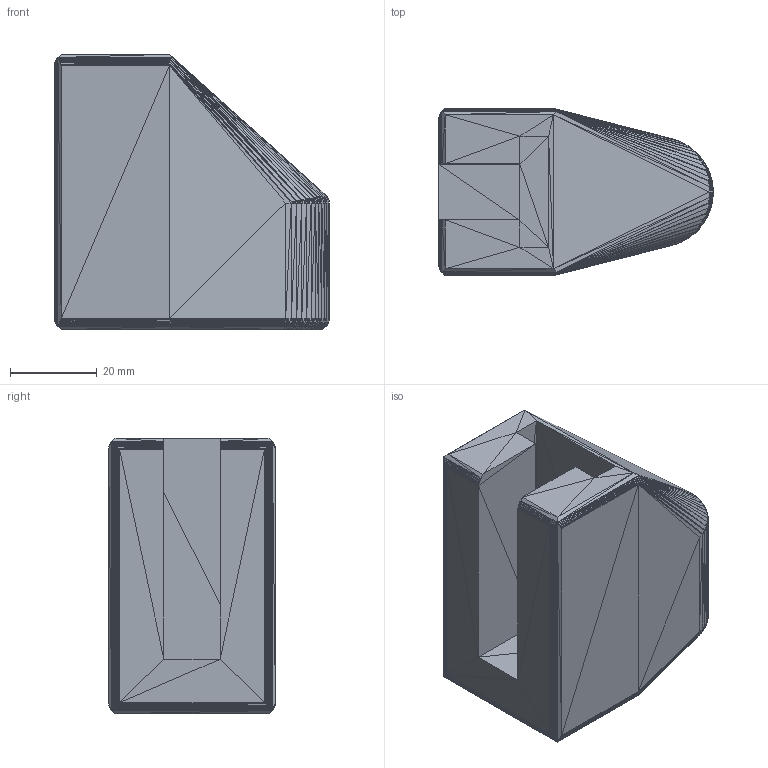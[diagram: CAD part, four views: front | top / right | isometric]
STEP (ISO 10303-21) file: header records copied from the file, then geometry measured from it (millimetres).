
FILE_DESCRIPTION(('FreeCAD Model'),'2;1');
FILE_NAME('Open CASCADE Shape Model','2021-09-30T11:08:04',('Author'),( ''),'Open CASCADE STEP processor 7.4','FreeCAD','Unknown');
FILE_SCHEMA(('AUTOMOTIVE_DESIGN { 1 0 10303 214 1 1 1 1 }'));
Length unit declared in the file: millimetre
Products named in the file (1): BARBB_Buttpad001_(Solid)
Bounding box: 63.3 x 38.48 x 63.5 mm (x, y, z)
Volume: 93718.9 mm3; surface area: 17609.8 mm2
Topology: 1 solids, 1 shells, 1154 faces, 1731 edges, 579 vertices
Faces by surface type: plane 1154
Entity records: 43309 total; most frequent: CARTESIAN_POINT 8658, DIRECTION 5772, ORIENTED_EDGE 3462, LINE 3462, VECTOR 3462, PCURVE 3462, DEFINITIONAL_REPRESENTATION 3462, EDGE_CURVE 1731
